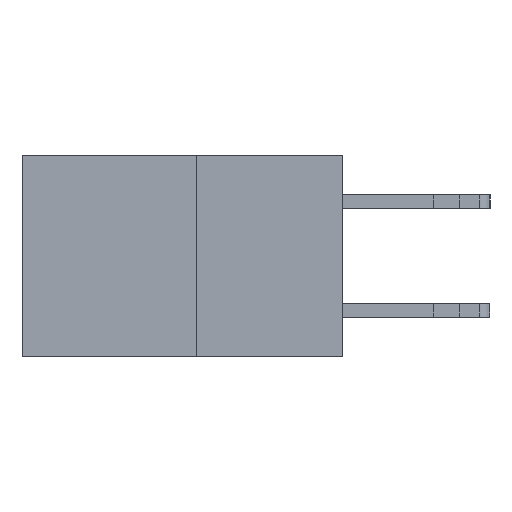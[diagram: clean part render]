
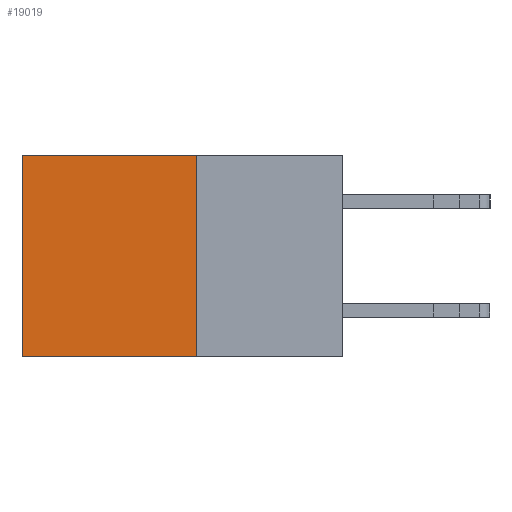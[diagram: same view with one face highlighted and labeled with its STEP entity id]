
A CAD part, left-side view. The second image highlights one B-rep face of the part: STEP entity #19019.
In plain terms, the highlighted planar face has unit normal (-1, 0, 0).
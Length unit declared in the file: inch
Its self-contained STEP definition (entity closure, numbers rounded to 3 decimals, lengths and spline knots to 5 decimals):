
#857 = ORIENTED_EDGE ( 'NONE', *, *, #15313, .T. ) ;
#1297 = EDGE_CURVE ( 'NONE', #2828, #16801, #10439, .T. ) ;
#2828 = VERTEX_POINT ( 'NONE', #9332 ) ;
#3728 = VECTOR ( 'NONE', #3879, 39.37008 ) ;
#3879 = DIRECTION ( 'NONE',  ( 0., 0., -1. ) ) ;
#4772 = FACE_OUTER_BOUND ( 'NONE', #10540, .T. ) ;
#4965 = CARTESIAN_POINT ( 'NONE',  ( 0.277, 0.27, -0.37 ) ) ;
#8069 = VERTEX_POINT ( 'NONE', #11846 ) ;
#8270 = VERTEX_POINT ( 'NONE', #12277 ) ;
#9007 = DIRECTION ( 'NONE',  ( 1., 0., 0. ) ) ;
#9015 = CARTESIAN_POINT ( 'NONE',  ( 0.277, 0.27, 0. ) ) ;
#9332 = CARTESIAN_POINT ( 'NONE',  ( 0.277, 0.27, 0. ) ) ;
#10439 = LINE ( 'NONE', #13345, #18771 ) ;
#10540 = EDGE_LOOP ( 'NONE', ( #857, #14891, #18003, #15504 ) ) ;
#10722 = LINE ( 'NONE', #4965, #19037 ) ;
#11846 = CARTESIAN_POINT ( 'NONE',  ( 0.277, 0.59, 0. ) ) ;
#12043 = VECTOR ( 'NONE', #15835, 39.37008 ) ;
#12277 = CARTESIAN_POINT ( 'NONE',  ( 0.277, 0.59, -0.37 ) ) ;
#12323 = CARTESIAN_POINT ( 'NONE',  ( 0.277, 0.27, -0.37 ) ) ;
#13345 = CARTESIAN_POINT ( 'NONE',  ( 0.277, 0.27, -0.37 ) ) ;
#13836 = LINE ( 'NONE', #20392, #3728 ) ;
#14891 = ORIENTED_EDGE ( 'NONE', *, *, #19377, .F. ) ;
#15313 = EDGE_CURVE ( 'NONE', #8069, #8270, #13836, .T. ) ;
#15504 = ORIENTED_EDGE ( 'NONE', *, *, #20369, .T. ) ;
#15755 = PLANE ( 'NONE',  #18257 ) ;
#15835 = DIRECTION ( 'NONE',  ( 0., 1., 0. ) ) ;
#16529 = LINE ( 'NONE', #9015, #12043 ) ;
#16801 = VERTEX_POINT ( 'NONE', #19904 ) ;
#18003 = ORIENTED_EDGE ( 'NONE', *, *, #1297, .F. ) ;
#18255 = DIRECTION ( 'NONE',  ( 0., 1., 0. ) ) ;
#18257 = AXIS2_PLACEMENT_3D ( 'NONE', #12323, #9007, #20572 ) ;
#18771 = VECTOR ( 'NONE', #20267, 39.37008 ) ;
#19019 = ADVANCED_FACE ( 'NONE', ( #4772 ), #15755, .F. ) ;
#19037 = VECTOR ( 'NONE', #18255, 39.37008 ) ;
#19377 = EDGE_CURVE ( 'NONE', #16801, #8270, #10722, .T. ) ;
#19904 = CARTESIAN_POINT ( 'NONE',  ( 0.277, 0.27, -0.37 ) ) ;
#20267 = DIRECTION ( 'NONE',  ( 0., 0., -1. ) ) ;
#20369 = EDGE_CURVE ( 'NONE', #2828, #8069, #16529, .T. ) ;
#20392 = CARTESIAN_POINT ( 'NONE',  ( 0.277, 0.59, -0.37 ) ) ;
#20572 = DIRECTION ( 'NONE',  ( 0., 0., -1. ) ) ;
